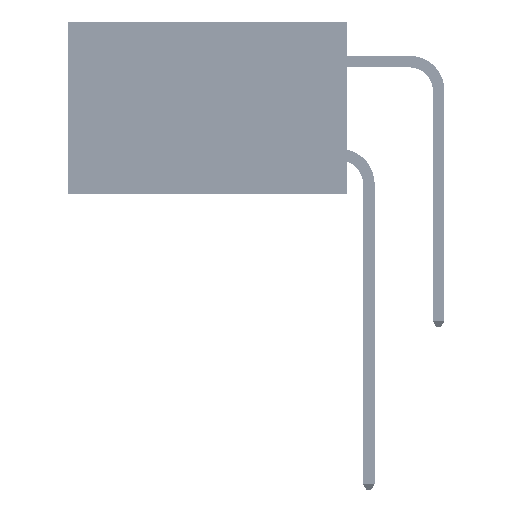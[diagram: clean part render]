
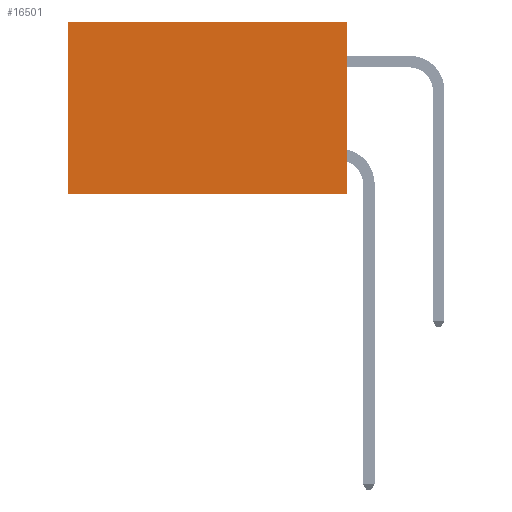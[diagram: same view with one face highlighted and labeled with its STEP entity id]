
A CAD part, left-side view. The second image highlights one B-rep face of the part: STEP entity #16501.
In plain terms, the highlighted planar face has unit normal (-1, 0, 0).
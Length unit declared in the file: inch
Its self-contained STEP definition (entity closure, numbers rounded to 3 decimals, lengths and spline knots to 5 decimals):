
#852 = EDGE_CURVE ( 'NONE', #10241, #5419, #52339, .T. ) ;
#4893 = EDGE_CURVE ( 'NONE', #5419, #9445, #24202, .T. ) ;
#5264 = ORIENTED_EDGE ( 'NONE', *, *, #18025, .F. ) ;
#5419 = VERTEX_POINT ( 'NONE', #43774 ) ;
#7481 = LINE ( 'NONE', #52262, #18365 ) ;
#9445 = VERTEX_POINT ( 'NONE', #16150 ) ;
#9969 = DIRECTION ( 'NONE',  ( 0., 0., -1. ) ) ;
#10241 = VERTEX_POINT ( 'NONE', #49330 ) ;
#13293 = VECTOR ( 'NONE', #48911, 39.37008 ) ;
#16150 = CARTESIAN_POINT ( 'NONE',  ( 0.2875, 0.6, -0.37 ) ) ;
#16501 = ADVANCED_FACE ( 'NONE', ( #38237 ), #18048, .F. ) ;
#18025 = EDGE_CURVE ( 'NONE', #52373, #9445, #7481, .T. ) ;
#18048 = PLANE ( 'NONE',  #37474 ) ;
#18365 = VECTOR ( 'NONE', #40100, 39.37008 ) ;
#20043 = VECTOR ( 'NONE', #32684, 39.37008 ) ;
#24202 = LINE ( 'NONE', #44873, #13293 ) ;
#24558 = CARTESIAN_POINT ( 'NONE',  ( 0.2875, 0., 0. ) ) ;
#25752 = CARTESIAN_POINT ( 'NONE',  ( 0.2875, 0., 0. ) ) ;
#29888 = VECTOR ( 'NONE', #41832, 39.37008 ) ;
#30009 = CARTESIAN_POINT ( 'NONE',  ( 0.2875, 0., -0.37 ) ) ;
#30063 = ORIENTED_EDGE ( 'NONE', *, *, #4893, .T. ) ;
#30322 = CARTESIAN_POINT ( 'NONE',  ( 0.2875, 0., 0. ) ) ;
#30924 = EDGE_LOOP ( 'NONE', ( #30063, #5264, #35554, #51215 ) ) ;
#31137 = LINE ( 'NONE', #25752, #29888 ) ;
#32684 = DIRECTION ( 'NONE',  ( 0., 1., 0. ) ) ;
#34139 = EDGE_CURVE ( 'NONE', #10241, #52373, #31137, .T. ) ;
#34363 = DIRECTION ( 'NONE',  ( 1., 0., 0. ) ) ;
#35554 = ORIENTED_EDGE ( 'NONE', *, *, #34139, .F. ) ;
#37474 = AXIS2_PLACEMENT_3D ( 'NONE', #30322, #34363, #9969 ) ;
#38237 = FACE_OUTER_BOUND ( 'NONE', #30924, .T. ) ;
#40100 = DIRECTION ( 'NONE',  ( 0., 1., 0. ) ) ;
#41832 = DIRECTION ( 'NONE',  ( 0., 0., -1. ) ) ;
#43774 = CARTESIAN_POINT ( 'NONE',  ( 0.2875, 0.6, 0. ) ) ;
#44873 = CARTESIAN_POINT ( 'NONE',  ( 0.2875, 0.6, 0. ) ) ;
#48911 = DIRECTION ( 'NONE',  ( 0., 0., -1. ) ) ;
#49330 = CARTESIAN_POINT ( 'NONE',  ( 0.2875, 0., 0. ) ) ;
#51215 = ORIENTED_EDGE ( 'NONE', *, *, #852, .T. ) ;
#52262 = CARTESIAN_POINT ( 'NONE',  ( 0.2875, 0., -0.37 ) ) ;
#52339 = LINE ( 'NONE', #24558, #20043 ) ;
#52373 = VERTEX_POINT ( 'NONE', #30009 ) ;
